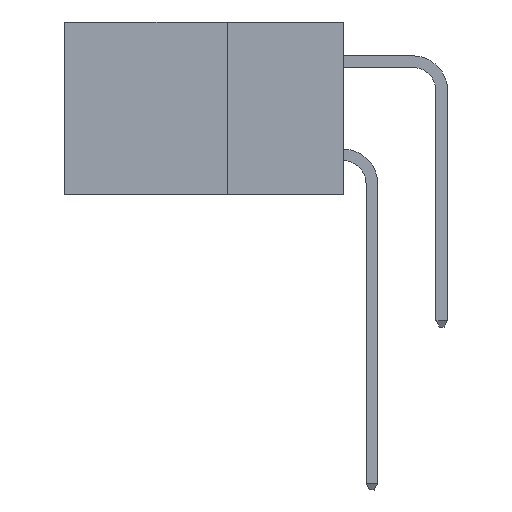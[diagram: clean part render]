
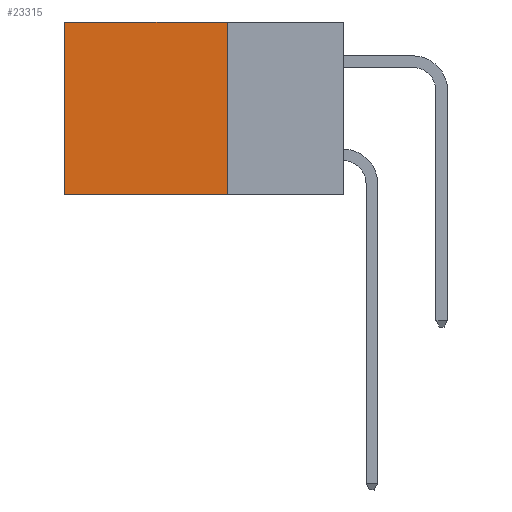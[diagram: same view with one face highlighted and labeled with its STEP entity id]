
A CAD part, left-side view. The second image highlights one B-rep face of the part: STEP entity #23315.
In plain terms, the highlighted planar face has unit normal (-1, 0, 0).
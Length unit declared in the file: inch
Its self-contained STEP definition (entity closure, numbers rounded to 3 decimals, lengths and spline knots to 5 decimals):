
#170 = VECTOR ( 'NONE', #19302, 39.37008 ) ;
#502 = DIRECTION ( 'NONE',  ( 1., 0., 0. ) ) ;
#842 = LINE ( 'NONE', #20660, #1791 ) ;
#918 = CARTESIAN_POINT ( 'NONE',  ( 0.298, 0.25, 0. ) ) ;
#1791 = VECTOR ( 'NONE', #2416, 39.37008 ) ;
#2327 = EDGE_CURVE ( 'NONE', #16271, #6764, #22511, .T. ) ;
#2416 = DIRECTION ( 'NONE',  ( 0., 1., 0. ) ) ;
#2678 = CARTESIAN_POINT ( 'NONE',  ( 0.298, 0.25, 0. ) ) ;
#4460 = VECTOR ( 'NONE', #16098, 39.37008 ) ;
#4537 = DIRECTION ( 'NONE',  ( 0., 0., -1. ) ) ;
#5078 = LINE ( 'NONE', #23524, #4460 ) ;
#5106 = ORIENTED_EDGE ( 'NONE', *, *, #15004, .F. ) ;
#5754 = VERTEX_POINT ( 'NONE', #11501 ) ;
#6138 = CARTESIAN_POINT ( 'NONE',  ( 0.298, 0.25, -0.37 ) ) ;
#6374 = PLANE ( 'NONE',  #8628 ) ;
#6764 = VERTEX_POINT ( 'NONE', #7754 ) ;
#7285 = ORIENTED_EDGE ( 'NONE', *, *, #12949, .T. ) ;
#7754 = CARTESIAN_POINT ( 'NONE',  ( 0.298, 0.6, 0. ) ) ;
#8628 = AXIS2_PLACEMENT_3D ( 'NONE', #16748, #502, #14754 ) ;
#9343 = VECTOR ( 'NONE', #4537, 39.37008 ) ;
#9656 = LINE ( 'NONE', #2678, #9343 ) ;
#10651 = FACE_OUTER_BOUND ( 'NONE', #19451, .T. ) ;
#11147 = ORIENTED_EDGE ( 'NONE', *, *, #16052, .F. ) ;
#11501 = CARTESIAN_POINT ( 'NONE',  ( 0.298, 0.6, -0.37 ) ) ;
#12725 = CARTESIAN_POINT ( 'NONE',  ( 0.298, 0.25, 0. ) ) ;
#12949 = EDGE_CURVE ( 'NONE', #6764, #5754, #5078, .T. ) ;
#14754 = DIRECTION ( 'NONE',  ( 0., 0., -1. ) ) ;
#15004 = EDGE_CURVE ( 'NONE', #21322, #5754, #842, .T. ) ;
#16052 = EDGE_CURVE ( 'NONE', #16271, #21322, #9656, .T. ) ;
#16098 = DIRECTION ( 'NONE',  ( 0., 0., -1. ) ) ;
#16271 = VERTEX_POINT ( 'NONE', #918 ) ;
#16748 = CARTESIAN_POINT ( 'NONE',  ( 0.298, 0.25, 0. ) ) ;
#19302 = DIRECTION ( 'NONE',  ( 0., 1., 0. ) ) ;
#19451 = EDGE_LOOP ( 'NONE', ( #7285, #5106, #11147, #20439 ) ) ;
#20439 = ORIENTED_EDGE ( 'NONE', *, *, #2327, .T. ) ;
#20660 = CARTESIAN_POINT ( 'NONE',  ( 0.298, 0.25, -0.37 ) ) ;
#21322 = VERTEX_POINT ( 'NONE', #6138 ) ;
#22511 = LINE ( 'NONE', #12725, #170 ) ;
#23315 = ADVANCED_FACE ( 'NONE', ( #10651 ), #6374, .F. ) ;
#23524 = CARTESIAN_POINT ( 'NONE',  ( 0.298, 0.6, 0. ) ) ;
